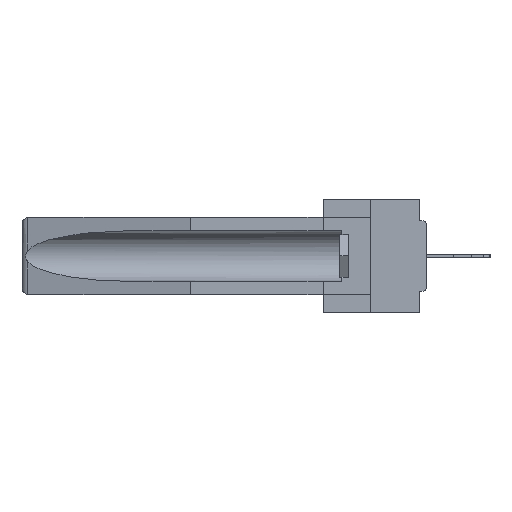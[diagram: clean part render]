
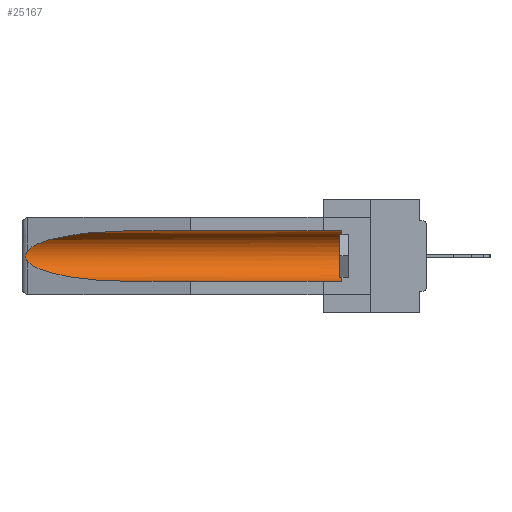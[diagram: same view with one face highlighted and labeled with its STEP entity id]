
A CAD part, left-side view. The second image highlights one B-rep face of the part: STEP entity #25167.
In plain terms, the highlighted cylindrical face has radius 2.857 mm (diameter 5.715 mm), a partial arc.
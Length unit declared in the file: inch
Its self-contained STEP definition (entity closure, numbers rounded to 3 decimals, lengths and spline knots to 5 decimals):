
#402 = CARTESIAN_POINT ( 'NONE',  ( 0.155, -0.30754, -0.1715 ) ) ;
#456 = CARTESIAN_POINT ( 'NONE',  ( 0.155, -0.30754, -0.284 ) ) ;
#1693 = ORIENTED_EDGE ( 'NONE', *, *, #16851, .T. ) ;
#2425 = VERTEX_POINT ( 'NONE', #31645 ) ;
#2570 = EDGE_LOOP ( 'NONE', ( #1693, #4681, #20921, #27215, #12697, #25694 ) ) ;
#3679 = EDGE_CURVE ( 'NONE', #23562, #26718, #21955, .T. ) ;
#4681 = ORIENTED_EDGE ( 'NONE', *, *, #3679, .T. ) ;
#5080 = CARTESIAN_POINT ( 'NONE',  ( 0.21114, 1.30732, -0.059 ) ) ;
#5139 = CARTESIAN_POINT ( 'NONE',  ( 0.155, 1.07973, -0.284 ) ) ;
#5388 = CARTESIAN_POINT ( 'NONE',  ( 0.155, 1.07973, -0.284 ) ) ;
#5966 = LINE ( 'NONE', #456, #23044 ) ;
#7324 = CARTESIAN_POINT ( 'NONE',  ( 0.2673, 1.53269, -0.17917 ) ) ;
#8046 = CARTESIAN_POINT ( 'NONE',  ( 0.26537, 1.52718, -0.19328 ) ) ;
#8271 = CARTESIAN_POINT ( 'NONE',  ( 0.25451, 1.48313, -0.09465 ) ) ;
#8583 = EDGE_CURVE ( 'NONE', #28945, #22946, #5966, .T. ) ;
#9159 = CARTESIAN_POINT ( 'NONE',  ( 0.26537, 1.52718, -0.14972 ) ) ;
#9290 = CARTESIAN_POINT ( 'NONE',  ( 0.2673, 1.5327, -0.16383 ) ) ;
#9464 = CARTESIAN_POINT ( 'NONE',  ( 0.2675, 1.53308, -0.17534 ) ) ;
#9567 = CARTESIAN_POINT ( 'NONE',  ( 0.155, 0.126, -0.059 ) ) ;
#10392 = CARTESIAN_POINT ( 'NONE',  ( 0.25451, 1.48313, -0.24835 ) ) ;
#11275 = DIRECTION ( 'NONE',  ( 0., 1., 0. ) ) ;
#11613 = EDGE_CURVE ( 'NONE', #32104, #2425, #28614, .T. ) ;
#12697 = ORIENTED_EDGE ( 'NONE', *, *, #34212, .T. ) ;
#13949 = FACE_OUTER_BOUND ( 'NONE', #2570, .T. ) ;
#13955 =( BOUNDED_CURVE ( )  B_SPLINE_CURVE ( 3, ( #35163, #5080, #8271, #15981 ),
 .UNSPECIFIED., .F., .T. ) 
 B_SPLINE_CURVE_WITH_KNOTS ( ( 4, 4 ),
 ( 4.71239, 6.08839 ),
 .UNSPECIFIED. ) 
 CURVE ( )  GEOMETRIC_REPRESENTATION_ITEM ( )  RATIONAL_B_SPLINE_CURVE ( ( 1., 0.848, 0.848, 1. ) ) 
 REPRESENTATION_ITEM ( '' )  );
#14836 = CARTESIAN_POINT ( 'NONE',  ( 0.26655, 1.53094, -0.18657 ) ) ;
#15188 = CARTESIAN_POINT ( 'NONE',  ( 0.26537, 1.52718, -0.14972 ) ) ;
#15359 = CARTESIAN_POINT ( 'NONE',  ( 0.26597, 1.52961, -0.15275 ) ) ;
#15981 = CARTESIAN_POINT ( 'NONE',  ( 0.26537, 1.52718, -0.14972 ) ) ;
#16503 = AXIS2_PLACEMENT_3D ( 'NONE', #402, #11275, #19515 ) ;
#16653 = CYLINDRICAL_SURFACE ( 'NONE', #16503, 0.1125 ) ;
#16851 = EDGE_CURVE ( 'NONE', #2425, #23562, #13955, .T. ) ;
#16878 = DIRECTION ( 'NONE',  ( 0., 1., 0. ) ) ;
#17313 = DIRECTION ( 'NONE',  ( 0., 1., 0. ) ) ;
#17526 = CARTESIAN_POINT ( 'NONE',  ( 0.26597, 1.5296, -0.19026 ) ) ;
#17901 = CARTESIAN_POINT ( 'NONE',  ( 0.155, 0.126, -0.1715 ) ) ;
#19065 = VECTOR ( 'NONE', #17313, 39.37008 ) ;
#19515 = DIRECTION ( 'NONE',  ( 0., 0., 1. ) ) ;
#20768 = DIRECTION ( 'NONE',  ( 0., -1., 0. ) ) ;
#20921 = ORIENTED_EDGE ( 'NONE', *, *, #34421, .T. ) ;
#21850 = CARTESIAN_POINT ( 'NONE',  ( 0.155, 0.126, -0.284 ) ) ;
#21955 = B_SPLINE_CURVE_WITH_KNOTS ( 'NONE', 3,
 ( #15188, #15359, #34039, #9290, #23112, #9464, #7324, #14836, #17526, #28473 ),
 .UNSPECIFIED., .F., .F.,
 ( 4, 2, 2, 2, 4 ),
 ( 0., 0.00029, 0.00058, 0.00087, 0.00117 ),
 .UNSPECIFIED. ) ;
#22538 = CARTESIAN_POINT ( 'NONE',  ( 0.155, -0.30754, -0.059 ) ) ;
#22946 = VERTEX_POINT ( 'NONE', #5139 ) ;
#23044 = VECTOR ( 'NONE', #16878, 39.37008 ) ;
#23112 = CARTESIAN_POINT ( 'NONE',  ( 0.2675, 1.53308, -0.16763 ) ) ;
#23562 = VERTEX_POINT ( 'NONE', #9159 ) ;
#23650 =( BOUNDED_CURVE ( )  B_SPLINE_CURVE ( 3, ( #8046, #10392, #29912, #5388 ),
 .UNSPECIFIED., .F., .T. ) 
 B_SPLINE_CURVE_WITH_KNOTS ( ( 4, 4 ),
 ( 0.1948, 1.5708 ),
 .UNSPECIFIED. ) 
 CURVE ( )  GEOMETRIC_REPRESENTATION_ITEM ( )  RATIONAL_B_SPLINE_CURVE ( ( 1., 0.848, 0.848, 1. ) ) 
 REPRESENTATION_ITEM ( '' )  );
#25167 = ADVANCED_FACE ( 'NONE', ( #13949 ), #16653, .F. ) ;
#25694 = ORIENTED_EDGE ( 'NONE', *, *, #11613, .T. ) ;
#26718 = VERTEX_POINT ( 'NONE', #33312 ) ;
#27215 = ORIENTED_EDGE ( 'NONE', *, *, #8583, .F. ) ;
#28473 = CARTESIAN_POINT ( 'NONE',  ( 0.26537, 1.52718, -0.19328 ) ) ;
#28614 = LINE ( 'NONE', #22538, #19065 ) ;
#28945 = VERTEX_POINT ( 'NONE', #21850 ) ;
#28968 = AXIS2_PLACEMENT_3D ( 'NONE', #17901, #20768, #34414 ) ;
#29912 = CARTESIAN_POINT ( 'NONE',  ( 0.21114, 1.30732, -0.284 ) ) ;
#31645 = CARTESIAN_POINT ( 'NONE',  ( 0.155, 1.07973, -0.059 ) ) ;
#32104 = VERTEX_POINT ( 'NONE', #9567 ) ;
#32992 = CIRCLE ( 'NONE', #28968, 0.1125 ) ;
#33312 = CARTESIAN_POINT ( 'NONE',  ( 0.26537, 1.52718, -0.19328 ) ) ;
#34039 = CARTESIAN_POINT ( 'NONE',  ( 0.26654, 1.53092, -0.15636 ) ) ;
#34212 = EDGE_CURVE ( 'NONE', #28945, #32104, #32992, .T. ) ;
#34414 = DIRECTION ( 'NONE',  ( 0., 0., 1. ) ) ;
#34421 = EDGE_CURVE ( 'NONE', #26718, #22946, #23650, .T. ) ;
#35163 = CARTESIAN_POINT ( 'NONE',  ( 0.155, 1.07973, -0.059 ) ) ;
